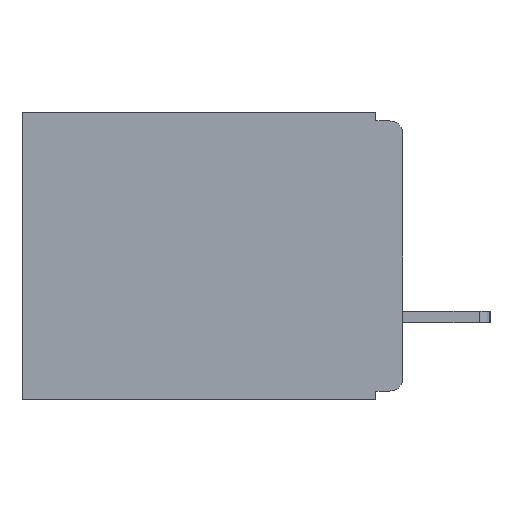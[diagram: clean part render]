
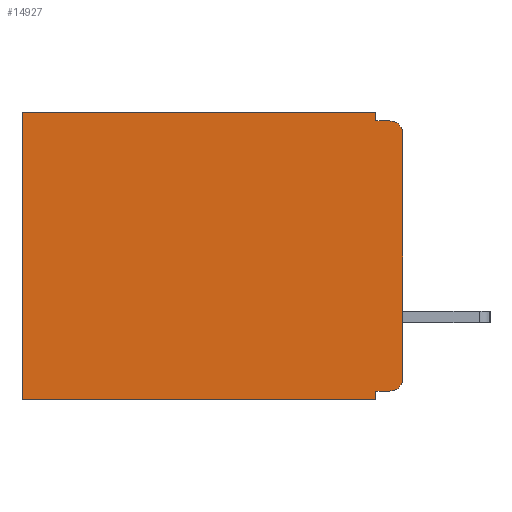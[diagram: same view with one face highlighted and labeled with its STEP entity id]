
A CAD part, left-side view. The second image highlights one B-rep face of the part: STEP entity #14927.
In plain terms, the highlighted planar face has unit normal (-1, 0, 0).
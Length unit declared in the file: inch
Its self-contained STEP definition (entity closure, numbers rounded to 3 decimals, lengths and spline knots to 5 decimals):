
#12 = DIRECTION ( 'NONE',  ( 0., 0., -1. ) ) ;
#977 = ORIENTED_EDGE ( 'NONE', *, *, #16115, .T. ) ;
#1433 = EDGE_CURVE ( 'NONE', #8173, #17374, #3660, .T. ) ;
#1696 = CARTESIAN_POINT ( 'NONE',  ( 0.3, 0., -0.32 ) ) ;
#1877 = CARTESIAN_POINT ( 'NONE',  ( 0.3, 0.437, -0.33 ) ) ;
#2091 = DIRECTION ( 'NONE',  ( 0., 0., -1. ) ) ;
#2538 = VECTOR ( 'NONE', #14044, 39.37008 ) ;
#2813 = VERTEX_POINT ( 'NONE', #9937 ) ;
#2856 = EDGE_CURVE ( 'NONE', #2813, #12400, #18476, .T. ) ;
#2909 = LINE ( 'NONE', #9616, #2538 ) ;
#3461 = VERTEX_POINT ( 'NONE', #5070 ) ;
#3660 = LINE ( 'NONE', #5814, #5505 ) ;
#3681 = VERTEX_POINT ( 'NONE', #6287 ) ;
#4105 = VERTEX_POINT ( 'NONE', #10094 ) ;
#4385 = EDGE_CURVE ( 'NONE', #3461, #14240, #9336, .T. ) ;
#4444 = VECTOR ( 'NONE', #4735, 39.37008 ) ;
#4467 = LINE ( 'NONE', #1696, #4444 ) ;
#4735 = DIRECTION ( 'NONE',  ( 0., 1., 0. ) ) ;
#4955 = EDGE_CURVE ( 'NONE', #4105, #14240, #6066, .T. ) ;
#5070 = CARTESIAN_POINT ( 'NONE',  ( 0.3, 0., -0.025 ) ) ;
#5156 = ORIENTED_EDGE ( 'NONE', *, *, #1433, .T. ) ;
#5262 = EDGE_CURVE ( 'NONE', #2813, #3681, #4467, .T. ) ;
#5461 = AXIS2_PLACEMENT_3D ( 'NONE', #10766, #6606, #12 ) ;
#5505 = VECTOR ( 'NONE', #13121, 39.37008 ) ;
#5578 = EDGE_CURVE ( 'NONE', #3681, #6221, #2909, .T. ) ;
#5814 = CARTESIAN_POINT ( 'NONE',  ( 0.3, 0., 0. ) ) ;
#6021 = VECTOR ( 'NONE', #9010, 39.37008 ) ;
#6066 = LINE ( 'NONE', #14738, #6021 ) ;
#6221 = VERTEX_POINT ( 'NONE', #12740 ) ;
#6287 = CARTESIAN_POINT ( 'NONE',  ( 0.3, 0.031, -0.32 ) ) ;
#6418 = LINE ( 'NONE', #8493, #9675 ) ;
#6606 = DIRECTION ( 'NONE',  ( -1., 0., 0. ) ) ;
#6803 = ORIENTED_EDGE ( 'NONE', *, *, #2856, .T. ) ;
#6921 = VECTOR ( 'NONE', #11974, 39.37008 ) ;
#6944 = LINE ( 'NONE', #13634, #6921 ) ;
#7239 = EDGE_CURVE ( 'NONE', #6221, #11691, #6418, .T. ) ;
#7763 = CARTESIAN_POINT ( 'NONE',  ( 0.3, 0., -0.305 ) ) ;
#8173 = VERTEX_POINT ( 'NONE', #14182 ) ;
#8348 = DIRECTION ( 'NONE',  ( 0., 1., 0. ) ) ;
#8453 = CARTESIAN_POINT ( 'NONE',  ( 0.3, 0.015, -0.01 ) ) ;
#8493 = CARTESIAN_POINT ( 'NONE',  ( 0.3, 0., -0.33 ) ) ;
#8932 = CARTESIAN_POINT ( 'NONE',  ( 0.3, 0.437, -0.33 ) ) ;
#9010 = DIRECTION ( 'NONE',  ( 0., -1., 0. ) ) ;
#9336 = CIRCLE ( 'NONE', #5461, 0.015 ) ;
#9616 = CARTESIAN_POINT ( 'NONE',  ( 0.3, 0.031, -0.33 ) ) ;
#9675 = VECTOR ( 'NONE', #8348, 39.37008 ) ;
#9689 = VECTOR ( 'NONE', #2091, 39.37008 ) ;
#9714 = CARTESIAN_POINT ( 'NONE',  ( 0.3, 0.437, 0. ) ) ;
#9728 = LINE ( 'NONE', #1877, #9689 ) ;
#9795 = EDGE_CURVE ( 'NONE', #3461, #12400, #16449, .T. ) ;
#9937 = CARTESIAN_POINT ( 'NONE',  ( 0.3, 0.015, -0.32 ) ) ;
#10094 = CARTESIAN_POINT ( 'NONE',  ( 0.3, 0.031, -0.01 ) ) ;
#10617 = ORIENTED_EDGE ( 'NONE', *, *, #4385, .T. ) ;
#10766 = CARTESIAN_POINT ( 'NONE',  ( 0.3, 0.015, -0.025 ) ) ;
#11121 = ORIENTED_EDGE ( 'NONE', *, *, #11856, .F. ) ;
#11691 = VERTEX_POINT ( 'NONE', #8932 ) ;
#11775 = ORIENTED_EDGE ( 'NONE', *, *, #5262, .F. ) ;
#11856 = EDGE_CURVE ( 'NONE', #8173, #4105, #6944, .T. ) ;
#11974 = DIRECTION ( 'NONE',  ( 0., 0., -1. ) ) ;
#12311 = CARTESIAN_POINT ( 'NONE',  ( 0.3, 0.015, -0.305 ) ) ;
#12400 = VERTEX_POINT ( 'NONE', #7763 ) ;
#12481 = AXIS2_PLACEMENT_3D ( 'NONE', #17789, #17761, #17756 ) ;
#12740 = CARTESIAN_POINT ( 'NONE',  ( 0.3, 0.031, -0.33 ) ) ;
#12825 = ORIENTED_EDGE ( 'NONE', *, *, #7239, .F. ) ;
#13074 = EDGE_LOOP ( 'NONE', ( #15302, #10617, #17585, #11121, #5156, #977, #12825, #14906, #11775, #6803 ) ) ;
#13121 = DIRECTION ( 'NONE',  ( 0., 1., 0. ) ) ;
#13305 = DIRECTION ( 'NONE',  ( -1., 0., 0. ) ) ;
#13384 = DIRECTION ( 'NONE',  ( 0., 0., -1. ) ) ;
#13634 = CARTESIAN_POINT ( 'NONE',  ( 0.3, 0.031, 0. ) ) ;
#14044 = DIRECTION ( 'NONE',  ( 0., 0., -1. ) ) ;
#14182 = CARTESIAN_POINT ( 'NONE',  ( 0.3, 0.031, 0. ) ) ;
#14240 = VERTEX_POINT ( 'NONE', #8453 ) ;
#14738 = CARTESIAN_POINT ( 'NONE',  ( 0.3, 0., -0.01 ) ) ;
#14906 = ORIENTED_EDGE ( 'NONE', *, *, #5578, .F. ) ;
#14927 = ADVANCED_FACE ( 'NONE', ( #15383 ), #17807, .F. ) ;
#15302 = ORIENTED_EDGE ( 'NONE', *, *, #9795, .F. ) ;
#15383 = FACE_OUTER_BOUND ( 'NONE', #13074, .T. ) ;
#15639 = CARTESIAN_POINT ( 'NONE',  ( 0.3, 0., -0.33 ) ) ;
#16115 = EDGE_CURVE ( 'NONE', #17374, #11691, #9728, .T. ) ;
#16194 = DIRECTION ( 'NONE',  ( 0., 0., -1. ) ) ;
#16336 = VECTOR ( 'NONE', #16194, 39.37008 ) ;
#16449 = LINE ( 'NONE', #15639, #16336 ) ;
#17374 = VERTEX_POINT ( 'NONE', #9714 ) ;
#17585 = ORIENTED_EDGE ( 'NONE', *, *, #4955, .F. ) ;
#17756 = DIRECTION ( 'NONE',  ( 0., 0., -1. ) ) ;
#17761 = DIRECTION ( 'NONE',  ( 1., 0., 0. ) ) ;
#17789 = CARTESIAN_POINT ( 'NONE',  ( 0.3, 0., -0.33 ) ) ;
#17807 = PLANE ( 'NONE',  #12481 ) ;
#17835 = AXIS2_PLACEMENT_3D ( 'NONE', #12311, #13305, #13384 ) ;
#18476 = CIRCLE ( 'NONE', #17835, 0.015 ) ;
